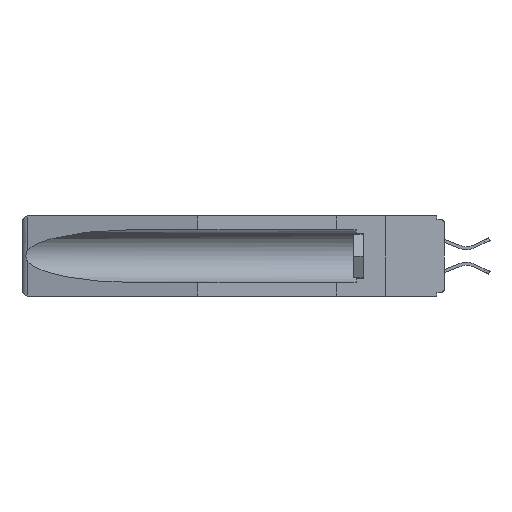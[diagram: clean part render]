
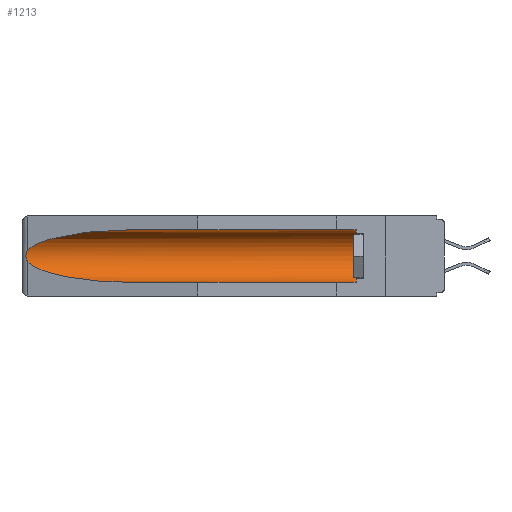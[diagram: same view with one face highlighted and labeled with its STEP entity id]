
A CAD part, left-side view. The second image highlights one B-rep face of the part: STEP entity #1213.
In plain terms, the highlighted cylindrical face has radius 2.857 mm (diameter 5.715 mm), a partial arc.
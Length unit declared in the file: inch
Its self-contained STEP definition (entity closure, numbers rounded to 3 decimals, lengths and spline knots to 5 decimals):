
#23 = CARTESIAN_POINT ( 'NONE',  ( 0.26654, 1.53092, -0.15636 ) ) ;
#101 = AXIS2_PLACEMENT_3D ( 'NONE', #4110, #20587, #7495 ) ;
#160 = EDGE_LOOP ( 'NONE', ( #5834, #16371, #15354, #7476, #15081, #12801 ) ) ;
#1213 = ADVANCED_FACE ( 'NONE', ( #4919 ), #7006, .F. ) ;
#1554 = CARTESIAN_POINT ( 'NONE',  ( 0.155, 1.07973, -0.059 ) ) ;
#2647 = DIRECTION ( 'NONE',  ( 0., 1., 0. ) ) ;
#2739 = VERTEX_POINT ( 'NONE', #10561 ) ;
#2945 = VERTEX_POINT ( 'NONE', #16130 ) ;
#3066 = CARTESIAN_POINT ( 'NONE',  ( 0.26655, 1.53094, -0.18657 ) ) ;
#3092 = CIRCLE ( 'NONE', #101, 0.1125 ) ;
#3118 = CARTESIAN_POINT ( 'NONE',  ( 0.155, -0.30754, -0.284 ) ) ;
#4110 = CARTESIAN_POINT ( 'NONE',  ( 0.155, 0.126, -0.1715 ) ) ;
#4387 = CARTESIAN_POINT ( 'NONE',  ( 0.155, -0.30754, -0.1715 ) ) ;
#4919 = FACE_OUTER_BOUND ( 'NONE', #160, .T. ) ;
#4963 = CARTESIAN_POINT ( 'NONE',  ( 0.26537, 1.52718, -0.14972 ) ) ;
#5834 = ORIENTED_EDGE ( 'NONE', *, *, #9762, .T. ) ;
#6352 = CARTESIAN_POINT ( 'NONE',  ( 0.25451, 1.48313, -0.09465 ) ) ;
#7006 = CYLINDRICAL_SURFACE ( 'NONE', #11717, 0.1125 ) ;
#7476 = ORIENTED_EDGE ( 'NONE', *, *, #12680, .F. ) ;
#7495 = DIRECTION ( 'NONE',  ( 0., 0., 1. ) ) ;
#7501 = DIRECTION ( 'NONE',  ( 0., 0., 1. ) ) ;
#7912 = CARTESIAN_POINT ( 'NONE',  ( 0.21114, 1.30732, -0.284 ) ) ;
#8232 = DIRECTION ( 'NONE',  ( 0., 1., 0. ) ) ;
#8245 = CARTESIAN_POINT ( 'NONE',  ( 0.2675, 1.53308, -0.16763 ) ) ;
#8996 = CARTESIAN_POINT ( 'NONE',  ( 0.155, 0.126, -0.284 ) ) ;
#9571 = VERTEX_POINT ( 'NONE', #11446 ) ;
#9591 = CARTESIAN_POINT ( 'NONE',  ( 0.155, 1.07973, -0.284 ) ) ;
#9653 = CARTESIAN_POINT ( 'NONE',  ( 0.26597, 1.5296, -0.19026 ) ) ;
#9762 = EDGE_CURVE ( 'NONE', #9571, #2739, #19074, .T. ) ;
#9847 = CARTESIAN_POINT ( 'NONE',  ( 0.2675, 1.53308, -0.17534 ) ) ;
#9919 = CARTESIAN_POINT ( 'NONE',  ( 0.26537, 1.52718, -0.19328 ) ) ;
#10144 = CARTESIAN_POINT ( 'NONE',  ( 0.26537, 1.52718, -0.19328 ) ) ;
#10561 = CARTESIAN_POINT ( 'NONE',  ( 0.26537, 1.52718, -0.14972 ) ) ;
#10811 =( BOUNDED_CURVE ( )  B_SPLINE_CURVE ( 3, ( #10981, #19491, #7912, #9591 ),
 .UNSPECIFIED., .F., .F. ) 
 B_SPLINE_CURVE_WITH_KNOTS ( ( 4, 4 ),
 ( 0.1948, 1.5708 ),
 .UNSPECIFIED. ) 
 CURVE ( )  GEOMETRIC_REPRESENTATION_ITEM ( )  RATIONAL_B_SPLINE_CURVE ( ( 1., 0.848, 0.848, 1. ) ) 
 REPRESENTATION_ITEM ( '' )  );
#10981 = CARTESIAN_POINT ( 'NONE',  ( 0.26537, 1.52718, -0.19328 ) ) ;
#11310 = CARTESIAN_POINT ( 'NONE',  ( 0.21114, 1.30732, -0.059 ) ) ;
#11381 = CARTESIAN_POINT ( 'NONE',  ( 0.26597, 1.52961, -0.15275 ) ) ;
#11446 = CARTESIAN_POINT ( 'NONE',  ( 0.155, 1.07973, -0.059 ) ) ;
#11717 = AXIS2_PLACEMENT_3D ( 'NONE', #4387, #12699, #7501 ) ;
#11911 = VECTOR ( 'NONE', #2647, 39.37008 ) ;
#12680 = EDGE_CURVE ( 'NONE', #14519, #15914, #16838, .T. ) ;
#12699 = DIRECTION ( 'NONE',  ( 0., 1., 0. ) ) ;
#12801 = ORIENTED_EDGE ( 'NONE', *, *, #17127, .T. ) ;
#13015 = CARTESIAN_POINT ( 'NONE',  ( 0.2673, 1.5327, -0.16383 ) ) ;
#13278 = B_SPLINE_CURVE_WITH_KNOTS ( 'NONE', 3,
 ( #19481, #11381, #23, #13015, #8245, #9847, #21251, #3066, #9653, #9919 ),
 .UNSPECIFIED., .F., .F.,
 ( 4, 2, 2, 2, 4 ),
 ( 0., 0.00029, 0.00058, 0.00087, 0.00117 ),
 .UNSPECIFIED. ) ;
#13853 = EDGE_CURVE ( 'NONE', #2739, #20946, #13278, .T. ) ;
#14279 = VECTOR ( 'NONE', #8232, 39.37008 ) ;
#14519 = VERTEX_POINT ( 'NONE', #8996 ) ;
#15081 = ORIENTED_EDGE ( 'NONE', *, *, #15318, .T. ) ;
#15318 = EDGE_CURVE ( 'NONE', #14519, #2945, #3092, .T. ) ;
#15354 = ORIENTED_EDGE ( 'NONE', *, *, #20633, .T. ) ;
#15914 = VERTEX_POINT ( 'NONE', #19060 ) ;
#16130 = CARTESIAN_POINT ( 'NONE',  ( 0.155, 0.126, -0.059 ) ) ;
#16371 = ORIENTED_EDGE ( 'NONE', *, *, #13853, .T. ) ;
#16838 = LINE ( 'NONE', #3118, #14279 ) ;
#17127 = EDGE_CURVE ( 'NONE', #2945, #9571, #20650, .T. ) ;
#17271 = CARTESIAN_POINT ( 'NONE',  ( 0.155, -0.30754, -0.059 ) ) ;
#19060 = CARTESIAN_POINT ( 'NONE',  ( 0.155, 1.07973, -0.284 ) ) ;
#19074 =( BOUNDED_CURVE ( )  B_SPLINE_CURVE ( 3, ( #1554, #11310, #6352, #4963 ),
 .UNSPECIFIED., .F., .F. ) 
 B_SPLINE_CURVE_WITH_KNOTS ( ( 4, 4 ),
 ( 4.71239, 6.08839 ),
 .UNSPECIFIED. ) 
 CURVE ( )  GEOMETRIC_REPRESENTATION_ITEM ( )  RATIONAL_B_SPLINE_CURVE ( ( 1., 0.848, 0.848, 1. ) ) 
 REPRESENTATION_ITEM ( '' )  );
#19481 = CARTESIAN_POINT ( 'NONE',  ( 0.26537, 1.52718, -0.14972 ) ) ;
#19491 = CARTESIAN_POINT ( 'NONE',  ( 0.25451, 1.48313, -0.24835 ) ) ;
#20587 = DIRECTION ( 'NONE',  ( 0., -1., 0. ) ) ;
#20633 = EDGE_CURVE ( 'NONE', #20946, #15914, #10811, .T. ) ;
#20650 = LINE ( 'NONE', #17271, #11911 ) ;
#20946 = VERTEX_POINT ( 'NONE', #10144 ) ;
#21251 = CARTESIAN_POINT ( 'NONE',  ( 0.2673, 1.53269, -0.17917 ) ) ;
